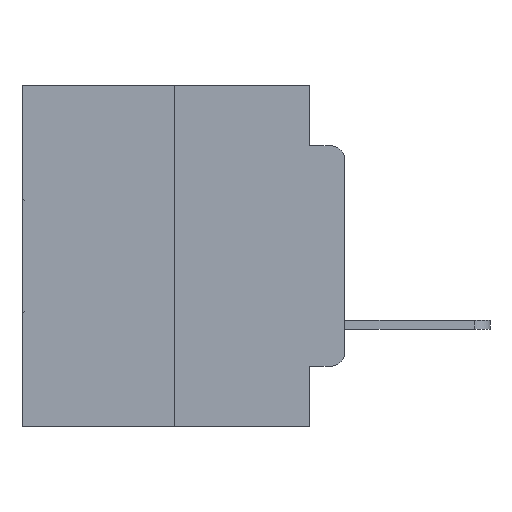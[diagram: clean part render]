
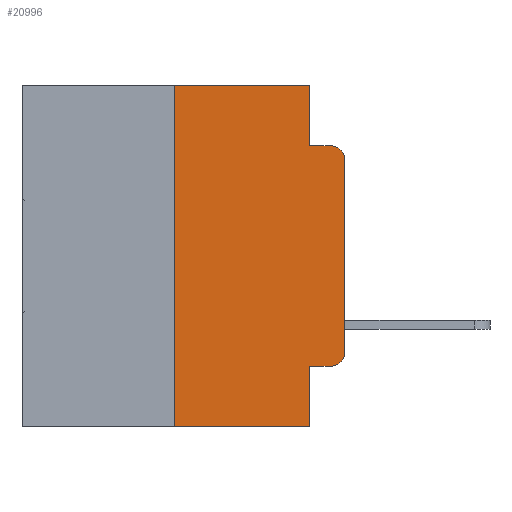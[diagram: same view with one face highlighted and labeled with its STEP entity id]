
A CAD part, left-side view. The second image highlights one B-rep face of the part: STEP entity #20996.
In plain terms, the highlighted planar face has unit normal (-1, 0, 0).
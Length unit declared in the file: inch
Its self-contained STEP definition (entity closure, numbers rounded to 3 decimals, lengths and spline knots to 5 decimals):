
#360 = CARTESIAN_POINT ( 'NONE',  ( 0., 0.25, 0. ) ) ;
#1059 = DIRECTION ( 'NONE',  ( 0., 0., -1. ) ) ;
#1149 = VERTEX_POINT ( 'NONE', #6163 ) ;
#1454 = AXIS2_PLACEMENT_3D ( 'NONE', #18544, #11425, #30467 ) ;
#2300 = LINE ( 'NONE', #4664, #26644 ) ;
#3706 = EDGE_CURVE ( 'NONE', #18345, #5121, #8165, .T. ) ;
#4113 = EDGE_LOOP ( 'NONE', ( #16363, #22236, #12343, #21778, #22994, #23715, #13098, #27146, #21482, #19046 ) ) ;
#4118 = DIRECTION ( 'NONE',  ( 0., -1., 0. ) ) ;
#4199 = DIRECTION ( 'NONE',  ( 0., 0., -1. ) ) ;
#4239 = VERTEX_POINT ( 'NONE', #16068 ) ;
#4550 = CARTESIAN_POINT ( 'NONE',  ( 0., 0.473, 0. ) ) ;
#4664 = CARTESIAN_POINT ( 'NONE',  ( 0., 0.051, -0.0885 ) ) ;
#4926 = VERTEX_POINT ( 'NONE', #360 ) ;
#5121 = VERTEX_POINT ( 'NONE', #20293 ) ;
#5494 = EDGE_CURVE ( 'NONE', #4926, #23152, #21730, .T. ) ;
#6011 = DIRECTION ( 'NONE',  ( 0., 0., 1. ) ) ;
#6163 = CARTESIAN_POINT ( 'NONE',  ( 0., 0.02, -0.4115 ) ) ;
#6191 = DIRECTION ( 'NONE',  ( 0., 0., -1. ) ) ;
#6224 = FACE_OUTER_BOUND ( 'NONE', #4113, .T. ) ;
#6244 = VECTOR ( 'NONE', #4118, 39.37008 ) ;
#6348 = DIRECTION ( 'NONE',  ( 0., 0., 1. ) ) ;
#6554 = VERTEX_POINT ( 'NONE', #19807 ) ;
#8165 = LINE ( 'NONE', #15933, #24783 ) ;
#8222 = CARTESIAN_POINT ( 'NONE',  ( 0., 0.051, 0. ) ) ;
#8302 = AXIS2_PLACEMENT_3D ( 'NONE', #12413, #17383, #1059 ) ;
#8450 = CARTESIAN_POINT ( 'NONE',  ( 0., 0.473, 0. ) ) ;
#8962 = LINE ( 'NONE', #30573, #27764 ) ;
#9279 = EDGE_CURVE ( 'NONE', #15038, #4239, #8962, .T. ) ;
#11032 = DIRECTION ( 'NONE',  ( 0., -1., 0. ) ) ;
#11425 = DIRECTION ( 'NONE',  ( -1., 0., 0. ) ) ;
#12300 = CARTESIAN_POINT ( 'NONE',  ( 0., 0.25, -0.5 ) ) ;
#12343 = ORIENTED_EDGE ( 'NONE', *, *, #28554, .F. ) ;
#12413 = CARTESIAN_POINT ( 'NONE',  ( 0., 0.02, -0.1085 ) ) ;
#12423 = AXIS2_PLACEMENT_3D ( 'NONE', #4550, #23460, #21185 ) ;
#12891 = EDGE_CURVE ( 'NONE', #5121, #26760, #14650, .T. ) ;
#12978 = EDGE_CURVE ( 'NONE', #15038, #4926, #29778, .T. ) ;
#13098 = ORIENTED_EDGE ( 'NONE', *, *, #9279, .T. ) ;
#13796 = LINE ( 'NONE', #26906, #16353 ) ;
#13984 = PLANE ( 'NONE',  #12423 ) ;
#14650 = CIRCLE ( 'NONE', #8302, 0.02 ) ;
#14769 = EDGE_CURVE ( 'NONE', #1149, #18345, #22706, .T. ) ;
#15038 = VERTEX_POINT ( 'NONE', #12300 ) ;
#15165 = VECTOR ( 'NONE', #4199, 39.37008 ) ;
#15583 = VERTEX_POINT ( 'NONE', #22362 ) ;
#15819 = CARTESIAN_POINT ( 'NONE',  ( 0., 0.051, 0. ) ) ;
#15863 = CARTESIAN_POINT ( 'NONE',  ( 0., 0.051, -0.4115 ) ) ;
#15882 = EDGE_CURVE ( 'NONE', #6554, #1149, #30227, .T. ) ;
#15933 = CARTESIAN_POINT ( 'NONE',  ( 0., 0., 0. ) ) ;
#16068 = CARTESIAN_POINT ( 'NONE',  ( 0., 0.051, -0.5 ) ) ;
#16353 = VECTOR ( 'NONE', #6191, 39.37008 ) ;
#16363 = ORIENTED_EDGE ( 'NONE', *, *, #3706, .T. ) ;
#17383 = DIRECTION ( 'NONE',  ( -1., 0., 0. ) ) ;
#17704 = VECTOR ( 'NONE', #11032, 39.37008 ) ;
#18345 = VERTEX_POINT ( 'NONE', #28584 ) ;
#18544 = CARTESIAN_POINT ( 'NONE',  ( 0., 0.02, -0.3915 ) ) ;
#19046 = ORIENTED_EDGE ( 'NONE', *, *, #14769, .T. ) ;
#19218 = DIRECTION ( 'NONE',  ( 0., -1., 0. ) ) ;
#19807 = CARTESIAN_POINT ( 'NONE',  ( 0., 0.051, -0.4115 ) ) ;
#20293 = CARTESIAN_POINT ( 'NONE',  ( 0., 0., -0.1085 ) ) ;
#20860 = CARTESIAN_POINT ( 'NONE',  ( 0., 0.02, -0.0885 ) ) ;
#20996 = ADVANCED_FACE ( 'NONE', ( #6224 ), #13984, .F. ) ;
#21185 = DIRECTION ( 'NONE',  ( 0., 0., -1. ) ) ;
#21482 = ORIENTED_EDGE ( 'NONE', *, *, #15882, .T. ) ;
#21730 = LINE ( 'NONE', #8450, #6244 ) ;
#21778 = ORIENTED_EDGE ( 'NONE', *, *, #29498, .F. ) ;
#22236 = ORIENTED_EDGE ( 'NONE', *, *, #12891, .T. ) ;
#22362 = CARTESIAN_POINT ( 'NONE',  ( 0., 0.051, -0.0885 ) ) ;
#22706 = CIRCLE ( 'NONE', #1454, 0.02 ) ;
#22994 = ORIENTED_EDGE ( 'NONE', *, *, #5494, .F. ) ;
#23152 = VERTEX_POINT ( 'NONE', #15819 ) ;
#23460 = DIRECTION ( 'NONE',  ( 1., 0., 0. ) ) ;
#23715 = ORIENTED_EDGE ( 'NONE', *, *, #12978, .F. ) ;
#24718 = EDGE_CURVE ( 'NONE', #6554, #4239, #13796, .T. ) ;
#24783 = VECTOR ( 'NONE', #6348, 39.37008 ) ;
#25135 = LINE ( 'NONE', #8222, #15165 ) ;
#26134 = DIRECTION ( 'NONE',  ( 0., -1., 0. ) ) ;
#26644 = VECTOR ( 'NONE', #26134, 39.37008 ) ;
#26760 = VERTEX_POINT ( 'NONE', #20860 ) ;
#26906 = CARTESIAN_POINT ( 'NONE',  ( 0., 0.051, 0. ) ) ;
#27146 = ORIENTED_EDGE ( 'NONE', *, *, #24718, .F. ) ;
#27154 = CARTESIAN_POINT ( 'NONE',  ( 0., 0.25, 0. ) ) ;
#27764 = VECTOR ( 'NONE', #19218, 39.37008 ) ;
#28554 = EDGE_CURVE ( 'NONE', #15583, #26760, #2300, .T. ) ;
#28584 = CARTESIAN_POINT ( 'NONE',  ( 0., 0., -0.3915 ) ) ;
#29007 = VECTOR ( 'NONE', #6011, 39.37008 ) ;
#29498 = EDGE_CURVE ( 'NONE', #23152, #15583, #25135, .T. ) ;
#29778 = LINE ( 'NONE', #27154, #29007 ) ;
#30227 = LINE ( 'NONE', #15863, #17704 ) ;
#30467 = DIRECTION ( 'NONE',  ( 0., 0., -1. ) ) ;
#30573 = CARTESIAN_POINT ( 'NONE',  ( 0., 0.473, -0.5 ) ) ;
